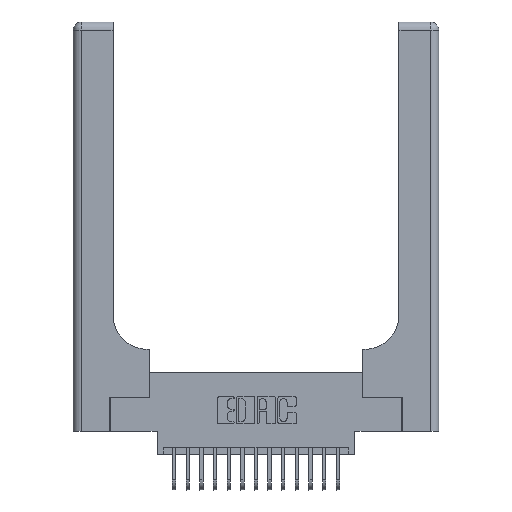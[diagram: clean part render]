
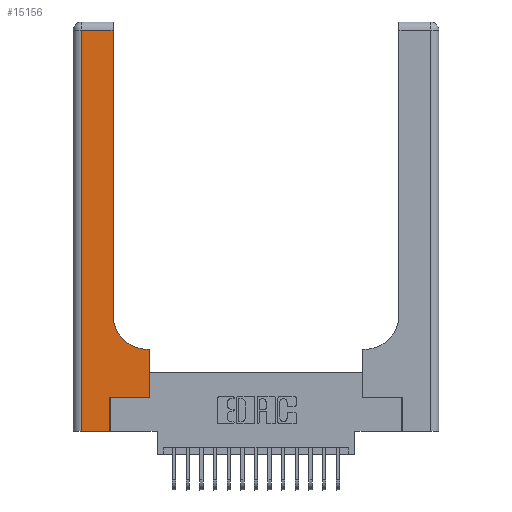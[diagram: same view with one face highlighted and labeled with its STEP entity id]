
A CAD part, top view. The second image highlights one B-rep face of the part: STEP entity #15156.
In plain terms, the highlighted planar face has unit normal (0, 0, 1).
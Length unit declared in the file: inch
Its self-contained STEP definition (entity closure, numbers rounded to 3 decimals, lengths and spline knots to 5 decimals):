
#680 = LINE ( 'NONE', #17413, #20761 ) ;
#1394 = VERTEX_POINT ( 'NONE', #2260 ) ;
#1486 = VERTEX_POINT ( 'NONE', #20258 ) ;
#1726 = EDGE_CURVE ( 'NONE', #3792, #17496, #19737, .T. ) ;
#1837 = VECTOR ( 'NONE', #12551, 39.37008 ) ;
#1943 = CARTESIAN_POINT ( 'NONE',  ( 0.06, 3., 0.37 ) ) ;
#2095 = ORIENTED_EDGE ( 'NONE', *, *, #12288, .T. ) ;
#2260 = CARTESIAN_POINT ( 'NONE',  ( 0.5415, 0.6, 0.37 ) ) ;
#2453 = CARTESIAN_POINT ( 'NONE',  ( 0.5585, 0.25, 0.37 ) ) ;
#2474 = ORIENTED_EDGE ( 'NONE', *, *, #9996, .T. ) ;
#2605 = ORIENTED_EDGE ( 'NONE', *, *, #7505, .T. ) ;
#3354 = ORIENTED_EDGE ( 'NONE', *, *, #5620, .T. ) ;
#3792 = VERTEX_POINT ( 'NONE', #10426 ) ;
#4020 = CARTESIAN_POINT ( 'NONE',  ( 0., 2.94, 0.37 ) ) ;
#4624 = CARTESIAN_POINT ( 'NONE',  ( 0.269, 0., 0.37 ) ) ;
#4777 = EDGE_CURVE ( 'NONE', #1486, #7738, #19854, .T. ) ;
#4829 = AXIS2_PLACEMENT_3D ( 'NONE', #17997, #8224, #19551 ) ;
#5174 = DIRECTION ( 'NONE',  ( 0., -1., 0. ) ) ;
#5410 = VERTEX_POINT ( 'NONE', #6197 ) ;
#5620 = EDGE_CURVE ( 'NONE', #5410, #3792, #15380, .T. ) ;
#5650 = FACE_OUTER_BOUND ( 'NONE', #18183, .T. ) ;
#6047 = EDGE_CURVE ( 'NONE', #1394, #1486, #17827, .T. ) ;
#6197 = CARTESIAN_POINT ( 'NONE',  ( 0.06, 2.94, 0.37 ) ) ;
#6675 = LINE ( 'NONE', #10882, #1837 ) ;
#6762 = VECTOR ( 'NONE', #13305, 39.37008 ) ;
#6902 = VECTOR ( 'NONE', #15615, 39.37008 ) ;
#6954 = ORIENTED_EDGE ( 'NONE', *, *, #11308, .T. ) ;
#7195 = PLANE ( 'NONE',  #15522 ) ;
#7490 = VERTEX_POINT ( 'NONE', #2453 ) ;
#7505 = EDGE_CURVE ( 'NONE', #18193, #7490, #11945, .T. ) ;
#7738 = VERTEX_POINT ( 'NONE', #7976 ) ;
#7976 = CARTESIAN_POINT ( 'NONE',  ( 0.2915, 2.94, 0.37 ) ) ;
#8224 = DIRECTION ( 'NONE',  ( 0., 0., -1. ) ) ;
#8885 = DIRECTION ( 'NONE',  ( 0., 0., -1. ) ) ;
#9017 = CARTESIAN_POINT ( 'NONE',  ( 0.269, 0.25, 0.37 ) ) ;
#9275 = DIRECTION ( 'NONE',  ( 0., 1., 0. ) ) ;
#9498 = CARTESIAN_POINT ( 'NONE',  ( 0.5585, 0.6, 0.37 ) ) ;
#9996 = EDGE_CURVE ( 'NONE', #14120, #1394, #6675, .T. ) ;
#10426 = CARTESIAN_POINT ( 'NONE',  ( 0.06, 0., 0.37 ) ) ;
#10805 = LINE ( 'NONE', #4020, #6902 ) ;
#10882 = CARTESIAN_POINT ( 'NONE',  ( 0.2915, 0.6, 0.37 ) ) ;
#10999 = VECTOR ( 'NONE', #5174, 39.37008 ) ;
#11308 = EDGE_CURVE ( 'NONE', #7490, #14120, #13631, .T. ) ;
#11945 = LINE ( 'NONE', #9017, #16318 ) ;
#12169 = ORIENTED_EDGE ( 'NONE', *, *, #6047, .T. ) ;
#12288 = EDGE_CURVE ( 'NONE', #17496, #18193, #680, .T. ) ;
#12551 = DIRECTION ( 'NONE',  ( -1., 0., 0. ) ) ;
#12679 = ORIENTED_EDGE ( 'NONE', *, *, #1726, .T. ) ;
#12937 = DIRECTION ( 'NONE',  ( 0., 1., 0. ) ) ;
#13180 = ORIENTED_EDGE ( 'NONE', *, *, #16711, .T. ) ;
#13305 = DIRECTION ( 'NONE',  ( 1., 0., 0. ) ) ;
#13631 = LINE ( 'NONE', #20872, #17418 ) ;
#14120 = VERTEX_POINT ( 'NONE', #9498 ) ;
#15156 = ADVANCED_FACE ( 'NONE', ( #5650 ), #7195, .F. ) ;
#15380 = LINE ( 'NONE', #1943, #10999 ) ;
#15383 = CARTESIAN_POINT ( 'NONE',  ( 0., 3., 0.37 ) ) ;
#15522 = AXIS2_PLACEMENT_3D ( 'NONE', #15383, #8885, #20171 ) ;
#15615 = DIRECTION ( 'NONE',  ( -1., 0., 0. ) ) ;
#16205 = VECTOR ( 'NONE', #18921, 39.37008 ) ;
#16318 = VECTOR ( 'NONE', #20354, 39.37008 ) ;
#16711 = EDGE_CURVE ( 'NONE', #7738, #5410, #10805, .T. ) ;
#17377 = CARTESIAN_POINT ( 'NONE',  ( 0.2915, 3., 0.37 ) ) ;
#17413 = CARTESIAN_POINT ( 'NONE',  ( 0.269, 0., 0.37 ) ) ;
#17418 = VECTOR ( 'NONE', #12937, 39.37008 ) ;
#17496 = VERTEX_POINT ( 'NONE', #4624 ) ;
#17827 = CIRCLE ( 'NONE', #4829, 0.25 ) ;
#17997 = CARTESIAN_POINT ( 'NONE',  ( 0.5415, 0.85, 0.37 ) ) ;
#18183 = EDGE_LOOP ( 'NONE', ( #19532, #13180, #3354, #12679, #2095, #2605, #6954, #2474, #12169 ) ) ;
#18193 = VERTEX_POINT ( 'NONE', #21040 ) ;
#18921 = DIRECTION ( 'NONE',  ( 0., 1., 0. ) ) ;
#19532 = ORIENTED_EDGE ( 'NONE', *, *, #4777, .T. ) ;
#19551 = DIRECTION ( 'NONE',  ( 1., 0., 0. ) ) ;
#19737 = LINE ( 'NONE', #21000, #6762 ) ;
#19854 = LINE ( 'NONE', #17377, #16205 ) ;
#20171 = DIRECTION ( 'NONE',  ( -1., 0., 0. ) ) ;
#20258 = CARTESIAN_POINT ( 'NONE',  ( 0.2915, 0.85, 0.37 ) ) ;
#20354 = DIRECTION ( 'NONE',  ( 1., 0., 0. ) ) ;
#20761 = VECTOR ( 'NONE', #9275, 39.37008 ) ;
#20872 = CARTESIAN_POINT ( 'NONE',  ( 0.5585, 0.25, 0.37 ) ) ;
#21000 = CARTESIAN_POINT ( 'NONE',  ( 0., 0., 0.37 ) ) ;
#21040 = CARTESIAN_POINT ( 'NONE',  ( 0.269, 0.25, 0.37 ) ) ;
